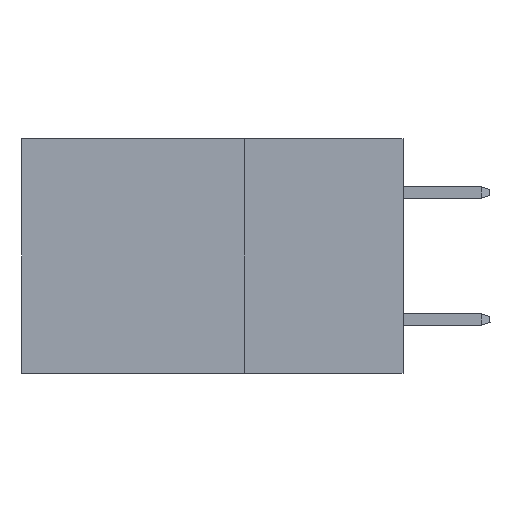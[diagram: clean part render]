
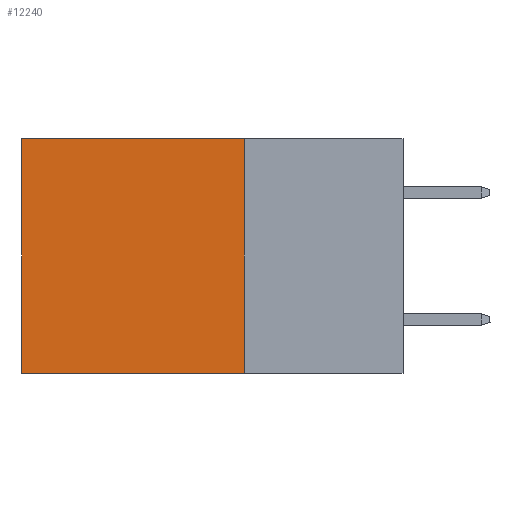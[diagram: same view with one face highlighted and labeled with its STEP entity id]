
A CAD part, left-side view. The second image highlights one B-rep face of the part: STEP entity #12240.
In plain terms, the highlighted planar face has unit normal (-1, 0, 0).
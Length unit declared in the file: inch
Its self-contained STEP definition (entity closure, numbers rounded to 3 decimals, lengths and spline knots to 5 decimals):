
#563 = EDGE_LOOP ( 'NONE', ( #11273, #7959, #12220, #11371 ) ) ;
#1191 = DIRECTION ( 'NONE',  ( 0., 0., -1. ) ) ;
#1443 = CARTESIAN_POINT ( 'NONE',  ( 0.2875, 0.6, 0. ) ) ;
#3513 = VERTEX_POINT ( 'NONE', #11507 ) ;
#3781 = DIRECTION ( 'NONE',  ( 0., 1., 0. ) ) ;
#3893 = VECTOR ( 'NONE', #3781, 39.37008 ) ;
#4590 = CARTESIAN_POINT ( 'NONE',  ( 0.2875, 0.25, 0. ) ) ;
#4788 = CARTESIAN_POINT ( 'NONE',  ( 0.2875, 0.25, 0. ) ) ;
#4951 = DIRECTION ( 'NONE',  ( 0., 0., -1. ) ) ;
#5543 = FACE_OUTER_BOUND ( 'NONE', #563, .T. ) ;
#5841 = CARTESIAN_POINT ( 'NONE',  ( 0.2875, 0.25, -0.37 ) ) ;
#6062 = AXIS2_PLACEMENT_3D ( 'NONE', #10063, #15058, #12488 ) ;
#7237 = VERTEX_POINT ( 'NONE', #5841 ) ;
#7643 = CARTESIAN_POINT ( 'NONE',  ( 0.2875, 0.25, -0.37 ) ) ;
#7959 = ORIENTED_EDGE ( 'NONE', *, *, #13393, .F. ) ;
#8340 = LINE ( 'NONE', #4788, #10564 ) ;
#8514 = LINE ( 'NONE', #1443, #10812 ) ;
#9174 = EDGE_CURVE ( 'NONE', #3513, #9688, #13879, .T. ) ;
#9481 = VERTEX_POINT ( 'NONE', #10017 ) ;
#9518 = VECTOR ( 'NONE', #12838, 39.37008 ) ;
#9688 = VERTEX_POINT ( 'NONE', #11714 ) ;
#9749 = LINE ( 'NONE', #7643, #3893 ) ;
#10017 = CARTESIAN_POINT ( 'NONE',  ( 0.2875, 0.6, -0.37 ) ) ;
#10063 = CARTESIAN_POINT ( 'NONE',  ( 0.2875, 0.25, 0. ) ) ;
#10144 = PLANE ( 'NONE',  #6062 ) ;
#10564 = VECTOR ( 'NONE', #1191, 39.37008 ) ;
#10812 = VECTOR ( 'NONE', #4951, 39.37008 ) ;
#11098 = EDGE_CURVE ( 'NONE', #9688, #9481, #8514, .T. ) ;
#11273 = ORIENTED_EDGE ( 'NONE', *, *, #11098, .T. ) ;
#11371 = ORIENTED_EDGE ( 'NONE', *, *, #9174, .T. ) ;
#11384 = EDGE_CURVE ( 'NONE', #3513, #7237, #8340, .T. ) ;
#11507 = CARTESIAN_POINT ( 'NONE',  ( 0.2875, 0.25, 0. ) ) ;
#11714 = CARTESIAN_POINT ( 'NONE',  ( 0.2875, 0.6, 0. ) ) ;
#12220 = ORIENTED_EDGE ( 'NONE', *, *, #11384, .F. ) ;
#12240 = ADVANCED_FACE ( 'NONE', ( #5543 ), #10144, .F. ) ;
#12488 = DIRECTION ( 'NONE',  ( 0., 0., -1. ) ) ;
#12838 = DIRECTION ( 'NONE',  ( 0., 1., 0. ) ) ;
#13393 = EDGE_CURVE ( 'NONE', #7237, #9481, #9749, .T. ) ;
#13879 = LINE ( 'NONE', #4590, #9518 ) ;
#15058 = DIRECTION ( 'NONE',  ( 1., 0., 0. ) ) ;
